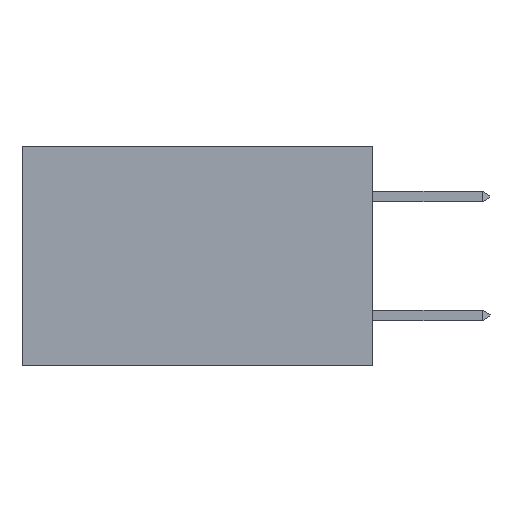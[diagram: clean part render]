
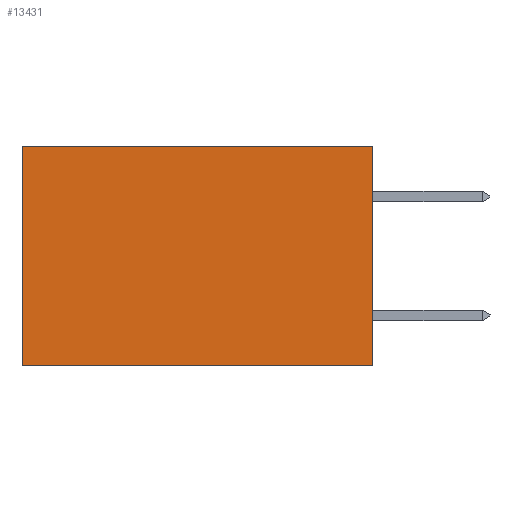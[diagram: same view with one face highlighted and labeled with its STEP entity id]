
A CAD part, left-side view. The second image highlights one B-rep face of the part: STEP entity #13431.
In plain terms, the highlighted planar face has unit normal (-1, 0, 0).
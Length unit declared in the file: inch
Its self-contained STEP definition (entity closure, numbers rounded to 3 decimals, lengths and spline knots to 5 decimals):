
#842 = DIRECTION ( 'NONE',  ( 0., 1., 0. ) ) ;
#1311 = LINE ( 'NONE', #15979, #21797 ) ;
#1495 = PLANE ( 'NONE',  #20169 ) ;
#2604 = LINE ( 'NONE', #8064, #12523 ) ;
#3688 = EDGE_CURVE ( 'NONE', #22698, #10331, #19887, .T. ) ;
#4516 = CARTESIAN_POINT ( 'NONE',  ( 0.277, 0.59, 0. ) ) ;
#4521 = ORIENTED_EDGE ( 'NONE', *, *, #18359, .F. ) ;
#5324 = CARTESIAN_POINT ( 'NONE',  ( 0.277, 0., 0. ) ) ;
#5561 = DIRECTION ( 'NONE',  ( 0., 0., -1. ) ) ;
#5818 = EDGE_LOOP ( 'NONE', ( #23580, #4521, #6665, #7339 ) ) ;
#6665 = ORIENTED_EDGE ( 'NONE', *, *, #13698, .F. ) ;
#7339 = ORIENTED_EDGE ( 'NONE', *, *, #3688, .T. ) ;
#8064 = CARTESIAN_POINT ( 'NONE',  ( 0.277, 0.59, -0.37 ) ) ;
#8096 = DIRECTION ( 'NONE',  ( 0., 0., -1. ) ) ;
#10015 = LINE ( 'NONE', #12817, #25157 ) ;
#10331 = VERTEX_POINT ( 'NONE', #4516 ) ;
#11528 = VERTEX_POINT ( 'NONE', #23676 ) ;
#12006 = DIRECTION ( 'NONE',  ( 0., 0., -1. ) ) ;
#12474 = VERTEX_POINT ( 'NONE', #24338 ) ;
#12523 = VECTOR ( 'NONE', #12006, 39.37008 ) ;
#12817 = CARTESIAN_POINT ( 'NONE',  ( 0.277, 0., -0.37 ) ) ;
#13431 = ADVANCED_FACE ( 'NONE', ( #14719 ), #1495, .F. ) ;
#13698 = EDGE_CURVE ( 'NONE', #22698, #12474, #1311, .T. ) ;
#14719 = FACE_OUTER_BOUND ( 'NONE', #5818, .T. ) ;
#15436 = CARTESIAN_POINT ( 'NONE',  ( 0.277, 0., -0.37 ) ) ;
#15979 = CARTESIAN_POINT ( 'NONE',  ( 0.277, 0., -0.37 ) ) ;
#17432 = DIRECTION ( 'NONE',  ( 1., 0., 0. ) ) ;
#18359 = EDGE_CURVE ( 'NONE', #12474, #11528, #10015, .T. ) ;
#19887 = LINE ( 'NONE', #5324, #23856 ) ;
#20169 = AXIS2_PLACEMENT_3D ( 'NONE', #15436, #17432, #5561 ) ;
#21797 = VECTOR ( 'NONE', #8096, 39.37008 ) ;
#22698 = VERTEX_POINT ( 'NONE', #23666 ) ;
#23580 = ORIENTED_EDGE ( 'NONE', *, *, #24734, .T. ) ;
#23666 = CARTESIAN_POINT ( 'NONE',  ( 0.277, 0., 0. ) ) ;
#23676 = CARTESIAN_POINT ( 'NONE',  ( 0.277, 0.59, -0.37 ) ) ;
#23856 = VECTOR ( 'NONE', #842, 39.37008 ) ;
#24338 = CARTESIAN_POINT ( 'NONE',  ( 0.277, 0., -0.37 ) ) ;
#24672 = DIRECTION ( 'NONE',  ( 0., 1., 0. ) ) ;
#24734 = EDGE_CURVE ( 'NONE', #10331, #11528, #2604, .T. ) ;
#25157 = VECTOR ( 'NONE', #24672, 39.37008 ) ;
